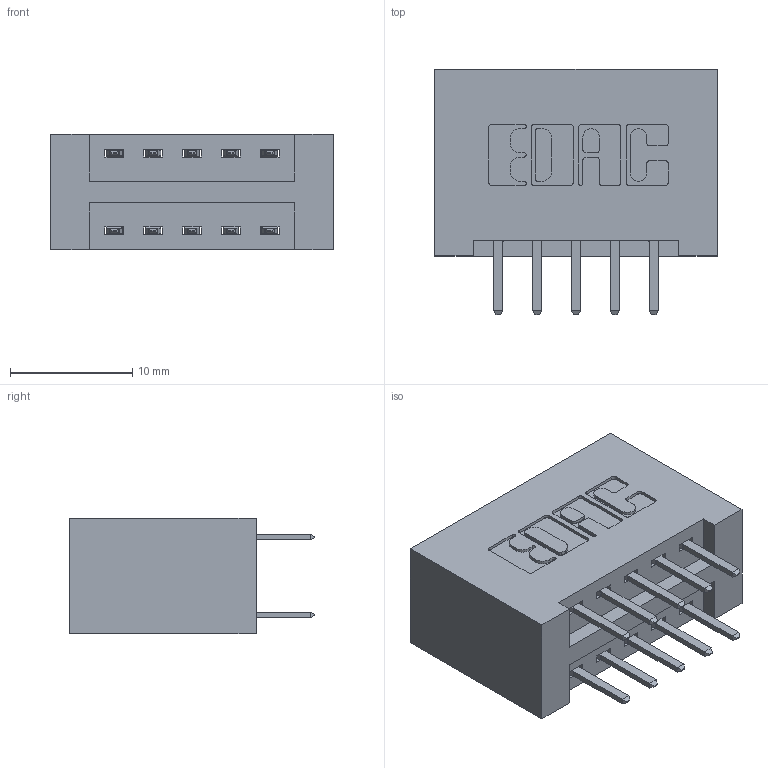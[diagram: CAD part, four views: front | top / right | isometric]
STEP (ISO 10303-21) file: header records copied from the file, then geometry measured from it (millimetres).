
FILE_DESCRIPTION (( 'STEP AP203' ), '1' );
FILE_NAME ('346-010-520-201.STEP', '2018-08-17T06:20:16', ( '' ), ( '' ), 'SwSTEP 2.0', 'SolidWorks 2016', '' );
FILE_SCHEMA (( 'CONFIG_CONTROL_DESIGN' ));
Length unit declared in the file: inch
Products named in the file (3): 345-292-001_345-293-120; 346-010-520-201; 346 Part_No Mounting Lugs
Assembly tree (11 placements, depth 2):
  346-010-520-201
    346 Part_No Mounting Lugs
    345-292-001_345-293-120  x10
Bounding box: 23.11 x 20.02 x 9.4 mm (x, y, z)
Volume: 2535.4 mm3; surface area: 3056.4 mm2
Topology: 11 solids, 11 shells, 674 faces, 1935 edges, 1262 vertices
Faces by surface type: plane 442, cylinder 232
Entity records: 8081 total; most frequent: CARTESIAN_POINT 1392, ORIENTED_EDGE 1314, DIRECTION 1261, EDGE_CURVE 657, VECTOR 509, LINE 509, VERTEX_POINT 434, AXIS2_PLACEMENT_3D 376
